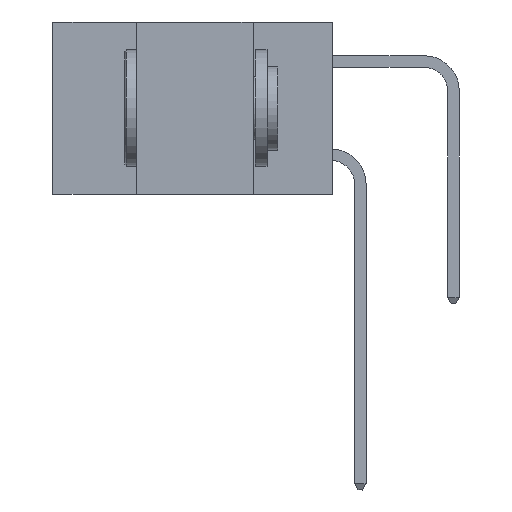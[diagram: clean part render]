
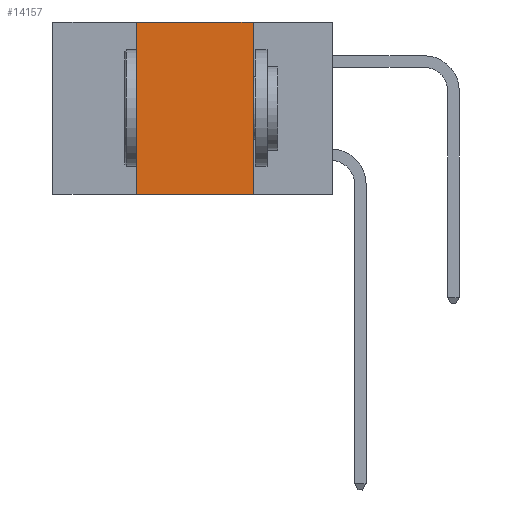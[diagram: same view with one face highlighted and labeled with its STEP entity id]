
A CAD part, left-side view. The second image highlights one B-rep face of the part: STEP entity #14157.
In plain terms, the highlighted planar face has unit normal (-1, 0, 0).
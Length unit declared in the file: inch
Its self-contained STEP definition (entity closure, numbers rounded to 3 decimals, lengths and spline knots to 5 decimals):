
#295 = ORIENTED_EDGE ( 'NONE', *, *, #6843, .F. ) ;
#381 = ORIENTED_EDGE ( 'NONE', *, *, #2829, .F. ) ;
#583 = VERTEX_POINT ( 'NONE', #1696 ) ;
#667 = DIRECTION ( 'NONE',  ( 0., 0., -1. ) ) ;
#1005 = CARTESIAN_POINT ( 'NONE',  ( 0., 0.42, 0. ) ) ;
#1035 = DIRECTION ( 'NONE',  ( 0., 0., -1. ) ) ;
#1696 = CARTESIAN_POINT ( 'NONE',  ( 0., 0.42, -0.37 ) ) ;
#2725 = EDGE_LOOP ( 'NONE', ( #381, #12419, #295, #8353 ) ) ;
#2829 = EDGE_CURVE ( 'NONE', #4172, #3352, #4098, .T. ) ;
#2955 = CARTESIAN_POINT ( 'NONE',  ( 0., 0.6, 0. ) ) ;
#3049 = DIRECTION ( 'NONE',  ( 0., -1., 0. ) ) ;
#3352 = VERTEX_POINT ( 'NONE', #5605 ) ;
#4098 = LINE ( 'NONE', #4113, #12682 ) ;
#4113 = CARTESIAN_POINT ( 'NONE',  ( 0., 0.17, 0. ) ) ;
#4172 = VERTEX_POINT ( 'NONE', #9391 ) ;
#5177 = VECTOR ( 'NONE', #3049, 39.37008 ) ;
#5605 = CARTESIAN_POINT ( 'NONE',  ( 0., 0.17, -0.37 ) ) ;
#6151 = VERTEX_POINT ( 'NONE', #1005 ) ;
#6641 = LINE ( 'NONE', #15607, #13177 ) ;
#6843 = EDGE_CURVE ( 'NONE', #583, #6151, #10478, .T. ) ;
#8000 = DIRECTION ( 'NONE',  ( 1., 0., 0. ) ) ;
#8353 = ORIENTED_EDGE ( 'NONE', *, *, #13022, .T. ) ;
#8362 = DIRECTION ( 'NONE',  ( 0., -1., 0. ) ) ;
#8801 = LINE ( 'NONE', #2955, #5177 ) ;
#9391 = CARTESIAN_POINT ( 'NONE',  ( 0., 0.17, 0. ) ) ;
#10133 = AXIS2_PLACEMENT_3D ( 'NONE', #10443, #8000, #667 ) ;
#10443 = CARTESIAN_POINT ( 'NONE',  ( 0., 0.6, 0. ) ) ;
#10478 = LINE ( 'NONE', #11303, #13329 ) ;
#11303 = CARTESIAN_POINT ( 'NONE',  ( 0., 0.42, 0. ) ) ;
#11703 = EDGE_CURVE ( 'NONE', #6151, #4172, #8801, .T. ) ;
#12419 = ORIENTED_EDGE ( 'NONE', *, *, #11703, .F. ) ;
#12682 = VECTOR ( 'NONE', #1035, 39.37008 ) ;
#13022 = EDGE_CURVE ( 'NONE', #583, #3352, #6641, .T. ) ;
#13177 = VECTOR ( 'NONE', #8362, 39.37008 ) ;
#13298 = DIRECTION ( 'NONE',  ( 0., 0., 1. ) ) ;
#13329 = VECTOR ( 'NONE', #13298, 39.37008 ) ;
#14157 = ADVANCED_FACE ( 'NONE', ( #15355 ), #15271, .F. ) ;
#15271 = PLANE ( 'NONE',  #10133 ) ;
#15355 = FACE_OUTER_BOUND ( 'NONE', #2725, .T. ) ;
#15607 = CARTESIAN_POINT ( 'NONE',  ( 0., 0.6, -0.37 ) ) ;
